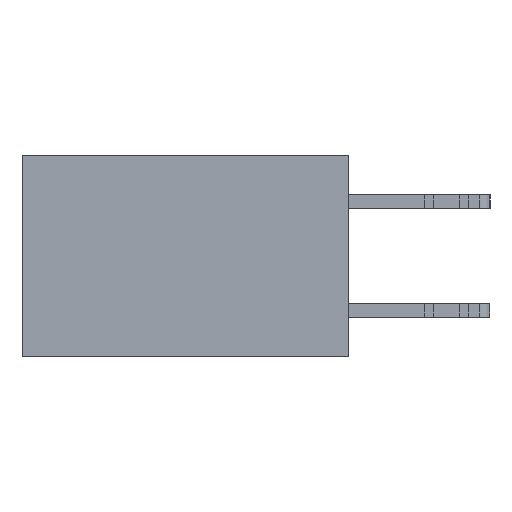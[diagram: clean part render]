
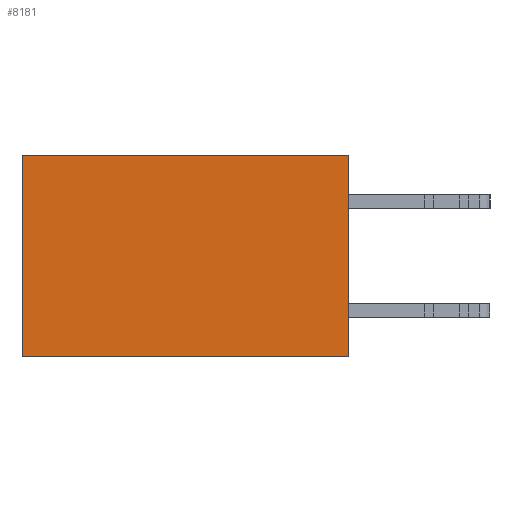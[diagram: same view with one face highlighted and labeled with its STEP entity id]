
A CAD part, left-side view. The second image highlights one B-rep face of the part: STEP entity #8181.
In plain terms, the highlighted planar face has unit normal (-1, 0, 0).
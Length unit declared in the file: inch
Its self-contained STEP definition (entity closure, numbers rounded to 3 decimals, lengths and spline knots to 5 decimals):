
#2067 = CARTESIAN_POINT ( 'NONE',  ( 0.298, 0., 0. ) ) ;
#2195 = EDGE_CURVE ( 'NONE', #12881, #30765, #23296, .T. ) ;
#2992 = VERTEX_POINT ( 'NONE', #19594 ) ;
#3825 = EDGE_LOOP ( 'NONE', ( #18512, #19018, #30695, #11877 ) ) ;
#6188 = CARTESIAN_POINT ( 'NONE',  ( 0.298, 0., 0. ) ) ;
#8181 = ADVANCED_FACE ( 'NONE', ( #29142 ), #12328, .F. ) ;
#9169 = CARTESIAN_POINT ( 'NONE',  ( 0.298, 0., 0. ) ) ;
#9281 = VERTEX_POINT ( 'NONE', #19092 ) ;
#10552 = DIRECTION ( 'NONE',  ( 0., 1., 0. ) ) ;
#10632 = AXIS2_PLACEMENT_3D ( 'NONE', #22517, #32607, #17467 ) ;
#11292 = DIRECTION ( 'NONE',  ( 0., 1., 0. ) ) ;
#11339 = VECTOR ( 'NONE', #17666, 39.37008 ) ;
#11877 = ORIENTED_EDGE ( 'NONE', *, *, #2195, .T. ) ;
#12328 = PLANE ( 'NONE',  #10632 ) ;
#12881 = VERTEX_POINT ( 'NONE', #9169 ) ;
#13884 = VECTOR ( 'NONE', #19972, 39.37008 ) ;
#15479 = LINE ( 'NONE', #2067, #13884 ) ;
#16427 = CARTESIAN_POINT ( 'NONE',  ( 0.298, 0., -0.37 ) ) ;
#17467 = DIRECTION ( 'NONE',  ( 0., 0., -1. ) ) ;
#17666 = DIRECTION ( 'NONE',  ( 0., 0., -1. ) ) ;
#17740 = LINE ( 'NONE', #16427, #30455 ) ;
#18512 = ORIENTED_EDGE ( 'NONE', *, *, #25953, .T. ) ;
#18950 = LINE ( 'NONE', #27817, #11339 ) ;
#19018 = ORIENTED_EDGE ( 'NONE', *, *, #26872, .F. ) ;
#19092 = CARTESIAN_POINT ( 'NONE',  ( 0.298, 0.6, -0.37 ) ) ;
#19594 = CARTESIAN_POINT ( 'NONE',  ( 0.298, 0., -0.37 ) ) ;
#19972 = DIRECTION ( 'NONE',  ( 0., 0., -1. ) ) ;
#22517 = CARTESIAN_POINT ( 'NONE',  ( 0.298, 0., 0. ) ) ;
#23296 = LINE ( 'NONE', #6188, #30034 ) ;
#25953 = EDGE_CURVE ( 'NONE', #30765, #9281, #18950, .T. ) ;
#26872 = EDGE_CURVE ( 'NONE', #2992, #9281, #17740, .T. ) ;
#27817 = CARTESIAN_POINT ( 'NONE',  ( 0.298, 0.6, 0. ) ) ;
#29142 = FACE_OUTER_BOUND ( 'NONE', #3825, .T. ) ;
#30034 = VECTOR ( 'NONE', #10552, 39.37008 ) ;
#30455 = VECTOR ( 'NONE', #11292, 39.37008 ) ;
#30695 = ORIENTED_EDGE ( 'NONE', *, *, #31741, .F. ) ;
#30765 = VERTEX_POINT ( 'NONE', #30858 ) ;
#30858 = CARTESIAN_POINT ( 'NONE',  ( 0.298, 0.6, 0. ) ) ;
#31741 = EDGE_CURVE ( 'NONE', #12881, #2992, #15479, .T. ) ;
#32607 = DIRECTION ( 'NONE',  ( 1., 0., 0. ) ) ;
